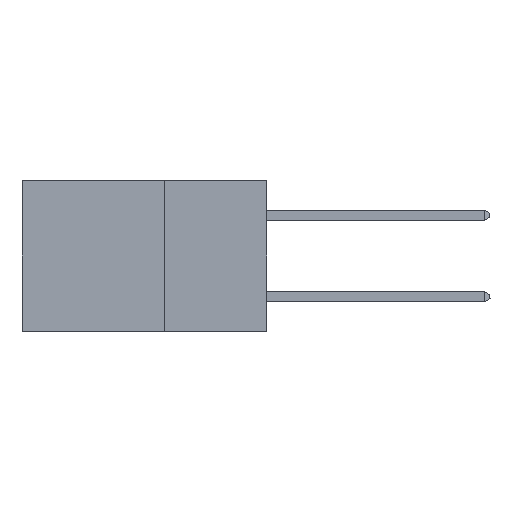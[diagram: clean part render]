
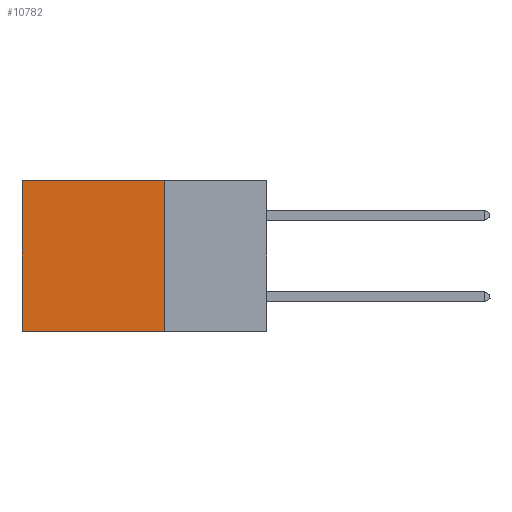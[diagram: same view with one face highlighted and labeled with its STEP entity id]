
A CAD part, left-side view. The second image highlights one B-rep face of the part: STEP entity #10782.
In plain terms, the highlighted planar face has unit normal (-1, 0, 0).
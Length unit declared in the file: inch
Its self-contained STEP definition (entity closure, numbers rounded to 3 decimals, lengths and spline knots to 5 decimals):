
#363 = CARTESIAN_POINT ( 'NONE',  ( 0.2875, 0.6, 0. ) ) ;
#713 = EDGE_CURVE ( 'NONE', #5803, #8259, #14936, .T. ) ;
#1837 = ORIENTED_EDGE ( 'NONE', *, *, #713, .F. ) ;
#2420 = CARTESIAN_POINT ( 'NONE',  ( 0.2875, 0.25, -0.37 ) ) ;
#3574 = CARTESIAN_POINT ( 'NONE',  ( 0.2875, 0.25, 0. ) ) ;
#4591 = EDGE_LOOP ( 'NONE', ( #5101, #19802, #1837, #16117 ) ) ;
#4668 = EDGE_CURVE ( 'NONE', #19323, #17521, #13162, .T. ) ;
#5101 = ORIENTED_EDGE ( 'NONE', *, *, #4668, .T. ) ;
#5803 = VERTEX_POINT ( 'NONE', #14250 ) ;
#6501 = AXIS2_PLACEMENT_3D ( 'NONE', #3574, #19152, #13935 ) ;
#6587 = CARTESIAN_POINT ( 'NONE',  ( 0.2875, 0.25, 0. ) ) ;
#7251 = CARTESIAN_POINT ( 'NONE',  ( 0.2875, 0.6, 0. ) ) ;
#7718 = DIRECTION ( 'NONE',  ( 0., 1., 0. ) ) ;
#8259 = VERTEX_POINT ( 'NONE', #14344 ) ;
#8612 = PLANE ( 'NONE',  #6501 ) ;
#9721 = EDGE_CURVE ( 'NONE', #8259, #17521, #10477, .T. ) ;
#10207 = EDGE_CURVE ( 'NONE', #5803, #19323, #17279, .T. ) ;
#10477 = LINE ( 'NONE', #2420, #19467 ) ;
#10782 = ADVANCED_FACE ( 'NONE', ( #14356 ), #8612, .F. ) ;
#12055 = CARTESIAN_POINT ( 'NONE',  ( 0.2875, 0.25, 0. ) ) ;
#12567 = DIRECTION ( 'NONE',  ( 0., 0., -1. ) ) ;
#12918 = CARTESIAN_POINT ( 'NONE',  ( 0.2875, 0.6, -0.37 ) ) ;
#13162 = LINE ( 'NONE', #363, #14812 ) ;
#13935 = DIRECTION ( 'NONE',  ( 0., 0., -1. ) ) ;
#14250 = CARTESIAN_POINT ( 'NONE',  ( 0.2875, 0.25, 0. ) ) ;
#14344 = CARTESIAN_POINT ( 'NONE',  ( 0.2875, 0.25, -0.37 ) ) ;
#14356 = FACE_OUTER_BOUND ( 'NONE', #4591, .T. ) ;
#14812 = VECTOR ( 'NONE', #12567, 39.37008 ) ;
#14936 = LINE ( 'NONE', #6587, #21761 ) ;
#15634 = VECTOR ( 'NONE', #20792, 39.37008 ) ;
#16117 = ORIENTED_EDGE ( 'NONE', *, *, #10207, .T. ) ;
#17279 = LINE ( 'NONE', #12055, #15634 ) ;
#17521 = VERTEX_POINT ( 'NONE', #12918 ) ;
#19152 = DIRECTION ( 'NONE',  ( 1., 0., 0. ) ) ;
#19323 = VERTEX_POINT ( 'NONE', #7251 ) ;
#19467 = VECTOR ( 'NONE', #7718, 39.37008 ) ;
#19802 = ORIENTED_EDGE ( 'NONE', *, *, #9721, .F. ) ;
#20354 = DIRECTION ( 'NONE',  ( 0., 0., -1. ) ) ;
#20792 = DIRECTION ( 'NONE',  ( 0., 1., 0. ) ) ;
#21761 = VECTOR ( 'NONE', #20354, 39.37008 ) ;
